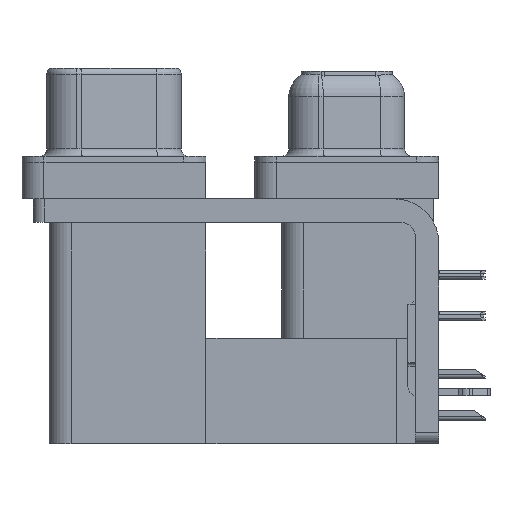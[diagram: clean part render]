
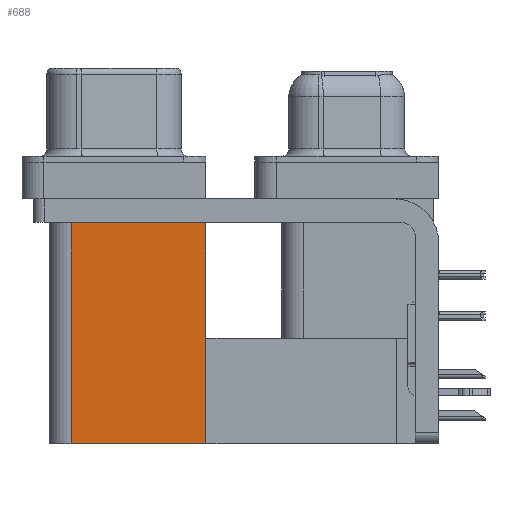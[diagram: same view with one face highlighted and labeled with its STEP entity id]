
A CAD part, left-side view. The second image highlights one B-rep face of the part: STEP entity #688.
In plain terms, the highlighted planar face has unit normal (-1, 0, 0).
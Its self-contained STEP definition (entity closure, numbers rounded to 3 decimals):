
#182 = LINE ( 'NONE', #3656, #35612 ) ;
#688 = ADVANCED_FACE ( 'NONE', ( #25469 ), #45943, .F. ) ;
#3656 = CARTESIAN_POINT ( 'NONE',  ( 3.765, 9.6, -19.2 ) ) ;
#3875 = DIRECTION ( 'NONE',  ( 1., 0., 0. ) ) ;
#7803 = EDGE_LOOP ( 'NONE', ( #34282, #28745, #16093, #42435 ) ) ;
#9351 = EDGE_CURVE ( 'NONE', #10339, #43049, #25022, .T. ) ;
#9361 = DIRECTION ( 'NONE',  ( 0., 1., 0. ) ) ;
#10339 = VERTEX_POINT ( 'NONE', #30473 ) ;
#10384 = CARTESIAN_POINT ( 'NONE',  ( 3.765, 9.6, -19.2 ) ) ;
#12154 = LINE ( 'NONE', #16312, #43663 ) ;
#12572 = EDGE_CURVE ( 'NONE', #10339, #22675, #182, .T. ) ;
#16054 = CARTESIAN_POINT ( 'NONE',  ( 3.765, 9.6, -2.5 ) ) ;
#16086 = VECTOR ( 'NONE', #42232, 1000. ) ;
#16093 = ORIENTED_EDGE ( 'NONE', *, *, #12572, .F. ) ;
#16312 = CARTESIAN_POINT ( 'NONE',  ( 3.765, 18.8, -19.2 ) ) ;
#16743 = VECTOR ( 'NONE', #9361, 1000. ) ;
#22208 = EDGE_CURVE ( 'NONE', #43049, #39059, #44693, .T. ) ;
#22675 = VERTEX_POINT ( 'NONE', #29321 ) ;
#25022 = LINE ( 'NONE', #43173, #16086 ) ;
#25469 = FACE_OUTER_BOUND ( 'NONE', #7803, .T. ) ;
#25624 = EDGE_CURVE ( 'NONE', #22675, #39059, #12154, .T. ) ;
#26543 = DIRECTION ( 'NONE',  ( 0., 0., 1. ) ) ;
#28500 = DIRECTION ( 'NONE',  ( 0., 0., -1. ) ) ;
#28745 = ORIENTED_EDGE ( 'NONE', *, *, #25624, .F. ) ;
#29321 = CARTESIAN_POINT ( 'NONE',  ( 3.765, 18.8, -19.2 ) ) ;
#30473 = CARTESIAN_POINT ( 'NONE',  ( 3.765, 9.6, -19.2 ) ) ;
#33851 = CARTESIAN_POINT ( 'NONE',  ( 3.765, 18.8, -2.5 ) ) ;
#34282 = ORIENTED_EDGE ( 'NONE', *, *, #22208, .T. ) ;
#35612 = VECTOR ( 'NONE', #39888, 1000. ) ;
#37710 = CARTESIAN_POINT ( 'NONE',  ( 3.765, 9.6, -2.5 ) ) ;
#37796 = AXIS2_PLACEMENT_3D ( 'NONE', #10384, #3875, #28500 ) ;
#39059 = VERTEX_POINT ( 'NONE', #33851 ) ;
#39888 = DIRECTION ( 'NONE',  ( 0., 1., 0. ) ) ;
#42232 = DIRECTION ( 'NONE',  ( 0., 0., 1. ) ) ;
#42435 = ORIENTED_EDGE ( 'NONE', *, *, #9351, .T. ) ;
#43049 = VERTEX_POINT ( 'NONE', #16054 ) ;
#43173 = CARTESIAN_POINT ( 'NONE',  ( 3.765, 9.6, -19.2 ) ) ;
#43663 = VECTOR ( 'NONE', #26543, 1000. ) ;
#44693 = LINE ( 'NONE', #37710, #16743 ) ;
#45943 = PLANE ( 'NONE',  #37796 ) ;
